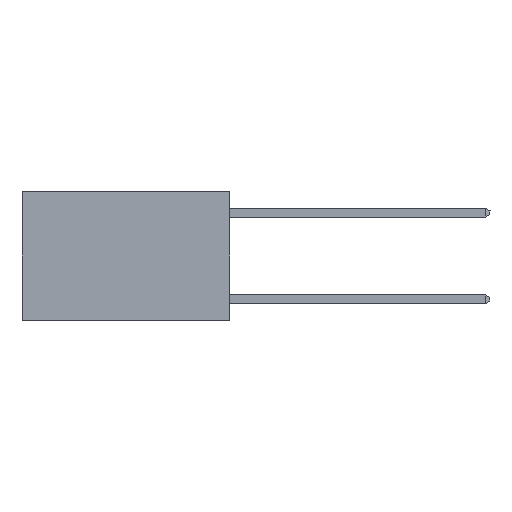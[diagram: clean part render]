
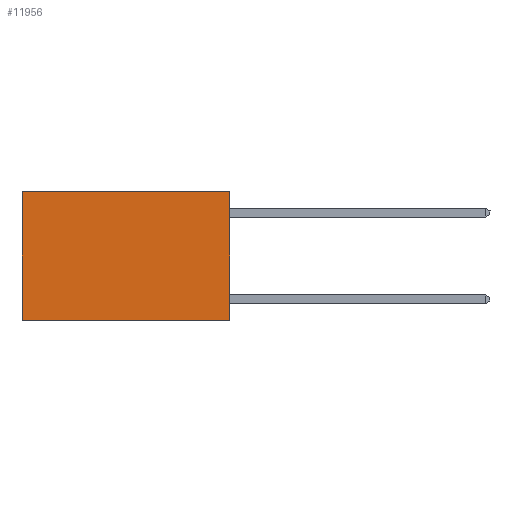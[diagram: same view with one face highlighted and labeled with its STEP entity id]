
A CAD part, left-side view. The second image highlights one B-rep face of the part: STEP entity #11956.
In plain terms, the highlighted planar face has unit normal (-1, 0, 0).
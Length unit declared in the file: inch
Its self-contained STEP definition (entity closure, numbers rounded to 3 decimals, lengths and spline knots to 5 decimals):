
#330 = ORIENTED_EDGE ( 'NONE', *, *, #13939, .T. ) ;
#938 = VERTEX_POINT ( 'NONE', #8355 ) ;
#1127 = DIRECTION ( 'NONE',  ( 0., 0., -1. ) ) ;
#1260 = CARTESIAN_POINT ( 'NONE',  ( 0.2625, 0., 0. ) ) ;
#2499 = AXIS2_PLACEMENT_3D ( 'NONE', #13229, #6410, #14345 ) ;
#2799 = VECTOR ( 'NONE', #13975, 39.37008 ) ;
#2800 = PLANE ( 'NONE',  #2499 ) ;
#3269 = CARTESIAN_POINT ( 'NONE',  ( 0.2625, 0.6, 0. ) ) ;
#4659 = CARTESIAN_POINT ( 'NONE',  ( 0.2625, 0., -0.37 ) ) ;
#4742 = ORIENTED_EDGE ( 'NONE', *, *, #10536, .F. ) ;
#4814 = CARTESIAN_POINT ( 'NONE',  ( 0.2625, 0., 0. ) ) ;
#4885 = LINE ( 'NONE', #15186, #10694 ) ;
#5117 = VERTEX_POINT ( 'NONE', #4659 ) ;
#5804 = FACE_OUTER_BOUND ( 'NONE', #7165, .T. ) ;
#5876 = CARTESIAN_POINT ( 'NONE',  ( 0.2625, 0.6, -0.37 ) ) ;
#6404 = LINE ( 'NONE', #15077, #8396 ) ;
#6410 = DIRECTION ( 'NONE',  ( 1., 0., 0. ) ) ;
#6673 = EDGE_CURVE ( 'NONE', #938, #5117, #13095, .T. ) ;
#7029 = VECTOR ( 'NONE', #10813, 39.37008 ) ;
#7165 = EDGE_LOOP ( 'NONE', ( #11517, #4742, #10242, #330 ) ) ;
#8327 = DIRECTION ( 'NONE',  ( 0., 1., 0. ) ) ;
#8355 = CARTESIAN_POINT ( 'NONE',  ( 0.2625, 0., 0. ) ) ;
#8396 = VECTOR ( 'NONE', #8327, 39.37008 ) ;
#10242 = ORIENTED_EDGE ( 'NONE', *, *, #6673, .F. ) ;
#10457 = VERTEX_POINT ( 'NONE', #5876 ) ;
#10536 = EDGE_CURVE ( 'NONE', #5117, #10457, #6404, .T. ) ;
#10694 = VECTOR ( 'NONE', #1127, 39.37008 ) ;
#10813 = DIRECTION ( 'NONE',  ( 0., 0., -1. ) ) ;
#11424 = VERTEX_POINT ( 'NONE', #3269 ) ;
#11517 = ORIENTED_EDGE ( 'NONE', *, *, #11762, .T. ) ;
#11762 = EDGE_CURVE ( 'NONE', #11424, #10457, #4885, .T. ) ;
#11956 = ADVANCED_FACE ( 'NONE', ( #5804 ), #2800, .F. ) ;
#12080 = LINE ( 'NONE', #4814, #2799 ) ;
#13095 = LINE ( 'NONE', #1260, #7029 ) ;
#13229 = CARTESIAN_POINT ( 'NONE',  ( 0.2625, 0., 0. ) ) ;
#13939 = EDGE_CURVE ( 'NONE', #938, #11424, #12080, .T. ) ;
#13975 = DIRECTION ( 'NONE',  ( 0., 1., 0. ) ) ;
#14345 = DIRECTION ( 'NONE',  ( 0., 0., -1. ) ) ;
#15077 = CARTESIAN_POINT ( 'NONE',  ( 0.2625, 0., -0.37 ) ) ;
#15186 = CARTESIAN_POINT ( 'NONE',  ( 0.2625, 0.6, 0. ) ) ;
